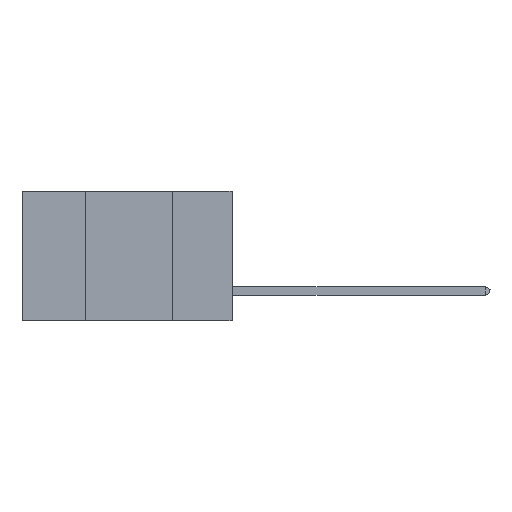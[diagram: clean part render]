
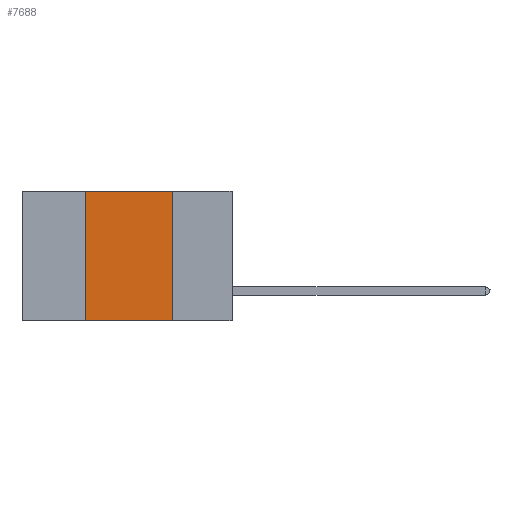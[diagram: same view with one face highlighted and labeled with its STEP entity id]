
A CAD part, left-side view. The second image highlights one B-rep face of the part: STEP entity #7688.
In plain terms, the highlighted planar face has unit normal (-1, 0, 0).
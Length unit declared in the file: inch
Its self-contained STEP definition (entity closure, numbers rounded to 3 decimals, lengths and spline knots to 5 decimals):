
#799 = VECTOR ( 'NONE', #15208, 39.37008 ) ;
#889 = EDGE_CURVE ( 'NONE', #10861, #31545, #40306, .T. ) ;
#1314 = CARTESIAN_POINT ( 'NONE',  ( 0., 0.6, 0. ) ) ;
#2590 = ORIENTED_EDGE ( 'NONE', *, *, #6772, .F. ) ;
#5020 = DIRECTION ( 'NONE',  ( 0., 0., 1. ) ) ;
#6700 = CARTESIAN_POINT ( 'NONE',  ( 0., 0.42, 0. ) ) ;
#6772 = EDGE_CURVE ( 'NONE', #31545, #24407, #17951, .T. ) ;
#7280 = CARTESIAN_POINT ( 'NONE',  ( 0., 0.17, 0. ) ) ;
#7688 = ADVANCED_FACE ( 'NONE', ( #25449 ), #17242, .F. ) ;
#7935 = CARTESIAN_POINT ( 'NONE',  ( 0., 0.17, 0. ) ) ;
#8628 = DIRECTION ( 'NONE',  ( 0., -1., 0. ) ) ;
#10624 = EDGE_LOOP ( 'NONE', ( #2590, #31170, #23899, #10787 ) ) ;
#10787 = ORIENTED_EDGE ( 'NONE', *, *, #12328, .T. ) ;
#10861 = VERTEX_POINT ( 'NONE', #15666 ) ;
#10901 = CARTESIAN_POINT ( 'NONE',  ( 0., 0.42, -0.37 ) ) ;
#11161 = DIRECTION ( 'NONE',  ( 1., 0., 0. ) ) ;
#11892 = CARTESIAN_POINT ( 'NONE',  ( 0., 0.6, -0.37 ) ) ;
#12328 = EDGE_CURVE ( 'NONE', #35114, #24407, #12744, .T. ) ;
#12744 = LINE ( 'NONE', #11892, #799 ) ;
#14426 = CARTESIAN_POINT ( 'NONE',  ( 0., 0.17, -0.37 ) ) ;
#14797 = LINE ( 'NONE', #6700, #29057 ) ;
#15208 = DIRECTION ( 'NONE',  ( 0., -1., 0. ) ) ;
#15234 = AXIS2_PLACEMENT_3D ( 'NONE', #1314, #11161, #20547 ) ;
#15666 = CARTESIAN_POINT ( 'NONE',  ( 0., 0.42, 0. ) ) ;
#17242 = PLANE ( 'NONE',  #15234 ) ;
#17951 = LINE ( 'NONE', #7935, #29775 ) ;
#19837 = EDGE_CURVE ( 'NONE', #35114, #10861, #14797, .T. ) ;
#20547 = DIRECTION ( 'NONE',  ( 0., 0., -1. ) ) ;
#23800 = DIRECTION ( 'NONE',  ( 0., 0., -1. ) ) ;
#23899 = ORIENTED_EDGE ( 'NONE', *, *, #19837, .F. ) ;
#24407 = VERTEX_POINT ( 'NONE', #14426 ) ;
#25449 = FACE_OUTER_BOUND ( 'NONE', #10624, .T. ) ;
#29057 = VECTOR ( 'NONE', #5020, 39.37008 ) ;
#29775 = VECTOR ( 'NONE', #23800, 39.37008 ) ;
#31170 = ORIENTED_EDGE ( 'NONE', *, *, #889, .F. ) ;
#31545 = VERTEX_POINT ( 'NONE', #7280 ) ;
#33752 = CARTESIAN_POINT ( 'NONE',  ( 0., 0.6, 0. ) ) ;
#35114 = VERTEX_POINT ( 'NONE', #10901 ) ;
#39806 = VECTOR ( 'NONE', #8628, 39.37008 ) ;
#40306 = LINE ( 'NONE', #33752, #39806 ) ;
